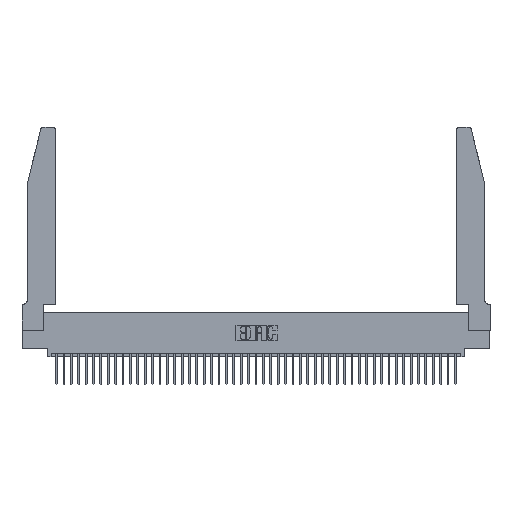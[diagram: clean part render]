
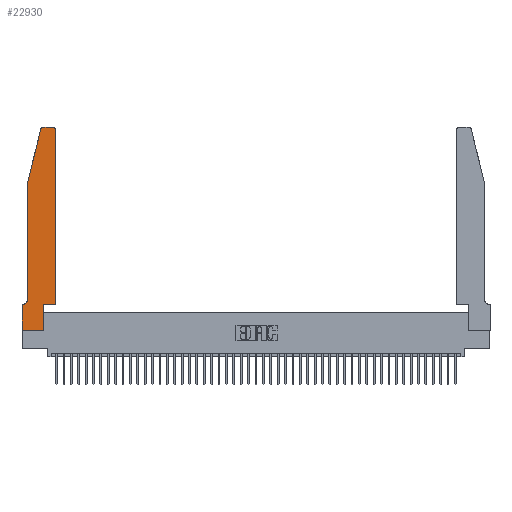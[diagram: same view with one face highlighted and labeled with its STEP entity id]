
A CAD part, top view. The second image highlights one B-rep face of the part: STEP entity #22930.
In plain terms, the highlighted planar face has unit normal (0, 0, 1).
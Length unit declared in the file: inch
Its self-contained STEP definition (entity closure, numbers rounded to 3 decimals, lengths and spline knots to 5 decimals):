
#414 = DIRECTION ( 'NONE',  ( 1., 0., 0. ) ) ;
#731 = VECTOR ( 'NONE', #16144, 39.37008 ) ;
#792 = CARTESIAN_POINT ( 'NONE',  ( 0., 0., 0.37 ) ) ;
#1232 = ORIENTED_EDGE ( 'NONE', *, *, #34104, .T. ) ;
#1706 = EDGE_CURVE ( 'NONE', #18084, #12142, #13387, .T. ) ;
#2321 = LINE ( 'NONE', #31248, #39360 ) ;
#2356 = VERTEX_POINT ( 'NONE', #45122 ) ;
#2507 = VECTOR ( 'NONE', #17822, 39.37008 ) ;
#2544 = DIRECTION ( 'NONE',  ( 0., 1., 0. ) ) ;
#3007 = DIRECTION ( 'NONE',  ( 0., 0., -1. ) ) ;
#3248 = VERTEX_POINT ( 'NONE', #18132 ) ;
#4471 = CARTESIAN_POINT ( 'NONE',  ( 0.0755, 2., 0.37 ) ) ;
#4486 = DIRECTION ( 'NONE',  ( 1., 0., 0. ) ) ;
#5032 = LINE ( 'NONE', #4471, #43030 ) ;
#5061 = DIRECTION ( 'NONE',  ( 0., 0., 1. ) ) ;
#5197 = VECTOR ( 'NONE', #2544, 39.37008 ) ;
#5380 = CARTESIAN_POINT ( 'NONE',  ( 0.0755, 0.42, 0.37 ) ) ;
#5472 = CIRCLE ( 'NONE', #22140, 0.07 ) ;
#6996 = VECTOR ( 'NONE', #44463, 39.37008 ) ;
#7797 = EDGE_CURVE ( 'NONE', #34003, #36792, #15695, .T. ) ;
#8155 = DIRECTION ( 'NONE',  ( 0., -1., 0. ) ) ;
#8232 = VERTEX_POINT ( 'NONE', #10209 ) ;
#9757 = CARTESIAN_POINT ( 'NONE',  ( 0.0755, 2., 0.37 ) ) ;
#9862 = CARTESIAN_POINT ( 'NONE',  ( 0., 0.35, 0.37 ) ) ;
#9913 = EDGE_CURVE ( 'NONE', #3248, #14087, #33858, .T. ) ;
#10167 = CARTESIAN_POINT ( 'NONE',  ( 0.4505, 2.72, 0.37 ) ) ;
#10209 = CARTESIAN_POINT ( 'NONE',  ( 0.2865, 0.35, 0.37 ) ) ;
#10376 = ORIENTED_EDGE ( 'NONE', *, *, #37209, .T. ) ;
#10499 = LINE ( 'NONE', #26812, #731 ) ;
#11829 = LINE ( 'NONE', #9757, #27554 ) ;
#12142 = VERTEX_POINT ( 'NONE', #45290 ) ;
#13387 = LINE ( 'NONE', #31409, #2507 ) ;
#13538 = DIRECTION ( 'NONE',  ( 1., 0., 0. ) ) ;
#14087 = VERTEX_POINT ( 'NONE', #10167 ) ;
#14396 = ORIENTED_EDGE ( 'NONE', *, *, #20613, .T. ) ;
#14770 = EDGE_CURVE ( 'NONE', #8232, #3248, #2321, .T. ) ;
#14876 = CARTESIAN_POINT ( 'NONE',  ( 0.2865, 0., 0.37 ) ) ;
#15167 = EDGE_LOOP ( 'NONE', ( #15466, #34423, #10376, #21123, #33890, #25610, #37212, #28919, #1232, #32279, #41601, #14396 ) ) ;
#15466 = ORIENTED_EDGE ( 'NONE', *, *, #33563, .T. ) ;
#15695 = LINE ( 'NONE', #792, #31376 ) ;
#16144 = DIRECTION ( 'NONE',  ( -1., 0., 0. ) ) ;
#17439 = DIRECTION ( 'NONE',  ( 0., -1., 0. ) ) ;
#17822 = DIRECTION ( 'NONE',  ( -1., 0., 0. ) ) ;
#17867 = AXIS2_PLACEMENT_3D ( 'NONE', #9862, #34877, #13538 ) ;
#18084 = VERTEX_POINT ( 'NONE', #20374 ) ;
#18132 = CARTESIAN_POINT ( 'NONE',  ( 0.4505, 0.35, 0.37 ) ) ;
#18966 = CARTESIAN_POINT ( 'NONE',  ( 0., 0., 0.37 ) ) ;
#19370 = CARTESIAN_POINT ( 'NONE',  ( 0.4205, 2.75, 0.37 ) ) ;
#19569 = CARTESIAN_POINT ( 'NONE',  ( 0.2865, 0.35, 0.37 ) ) ;
#19875 = AXIS2_PLACEMENT_3D ( 'NONE', #26706, #5061, #30272 ) ;
#20374 = CARTESIAN_POINT ( 'NONE',  ( 0.0055, 0.35, 0.37 ) ) ;
#20613 = EDGE_CURVE ( 'NONE', #14087, #37615, #25613, .T. ) ;
#21123 = ORIENTED_EDGE ( 'NONE', *, *, #28680, .T. ) ;
#22140 = AXIS2_PLACEMENT_3D ( 'NONE', #24723, #3007, #28285 ) ;
#22216 = DIRECTION ( 'NONE',  ( 0., 0., 1. ) ) ;
#22707 = FACE_OUTER_BOUND ( 'NONE', #15167, .T. ) ;
#22930 = ADVANCED_FACE ( 'NONE', ( #22707 ), #31381, .T. ) ;
#24165 = CIRCLE ( 'NONE', #19875, 0.03 ) ;
#24248 = DIRECTION ( 'NONE',  ( 1., 0., 0. ) ) ;
#24723 = CARTESIAN_POINT ( 'NONE',  ( 0.0055, 0.42, 0.37 ) ) ;
#25171 = EDGE_CURVE ( 'NONE', #25639, #18084, #5472, .T. ) ;
#25610 = ORIENTED_EDGE ( 'NONE', *, *, #1706, .T. ) ;
#25613 = CIRCLE ( 'NONE', #31285, 0.03 ) ;
#25639 = VERTEX_POINT ( 'NONE', #5380 ) ;
#26706 = CARTESIAN_POINT ( 'NONE',  ( 0.284, 2.72, 0.37 ) ) ;
#26812 = CARTESIAN_POINT ( 'NONE',  ( 0.2605, 2.75, 0.37 ) ) ;
#27554 = VECTOR ( 'NONE', #45360, 39.37008 ) ;
#28175 = VERTEX_POINT ( 'NONE', #30518 ) ;
#28285 = DIRECTION ( 'NONE',  ( -1., 0., 0. ) ) ;
#28680 = EDGE_CURVE ( 'NONE', #28175, #25639, #5032, .T. ) ;
#28919 = ORIENTED_EDGE ( 'NONE', *, *, #7797, .T. ) ;
#29690 = LINE ( 'NONE', #31951, #46134 ) ;
#30056 = EDGE_CURVE ( 'NONE', #33862, #2356, #24165, .T. ) ;
#30272 = DIRECTION ( 'NONE',  ( 1., 0., 0. ) ) ;
#30398 = EDGE_CURVE ( 'NONE', #12142, #34003, #29690, .T. ) ;
#30518 = CARTESIAN_POINT ( 'NONE',  ( 0.0755, 2., 0.37 ) ) ;
#31248 = CARTESIAN_POINT ( 'NONE',  ( 0.4505, 0.35, 0.37 ) ) ;
#31285 = AXIS2_PLACEMENT_3D ( 'NONE', #43341, #22216, #414 ) ;
#31376 = VECTOR ( 'NONE', #4486, 39.37008 ) ;
#31381 = PLANE ( 'NONE',  #17867 ) ;
#31409 = CARTESIAN_POINT ( 'NONE',  ( 0.0755, 0.35, 0.37 ) ) ;
#31951 = CARTESIAN_POINT ( 'NONE',  ( 0., 0., 0.37 ) ) ;
#32279 = ORIENTED_EDGE ( 'NONE', *, *, #14770, .T. ) ;
#33563 = EDGE_CURVE ( 'NONE', #37615, #33862, #10499, .T. ) ;
#33858 = LINE ( 'NONE', #41844, #5197 ) ;
#33862 = VERTEX_POINT ( 'NONE', #35580 ) ;
#33890 = ORIENTED_EDGE ( 'NONE', *, *, #25171, .T. ) ;
#34003 = VERTEX_POINT ( 'NONE', #18966 ) ;
#34104 = EDGE_CURVE ( 'NONE', #36792, #8232, #44915, .T. ) ;
#34423 = ORIENTED_EDGE ( 'NONE', *, *, #30056, .T. ) ;
#34877 = DIRECTION ( 'NONE',  ( 0., 0., 1. ) ) ;
#35580 = CARTESIAN_POINT ( 'NONE',  ( 0.284, 2.75, 0.37 ) ) ;
#36792 = VERTEX_POINT ( 'NONE', #14876 ) ;
#37209 = EDGE_CURVE ( 'NONE', #2356, #28175, #11829, .T. ) ;
#37212 = ORIENTED_EDGE ( 'NONE', *, *, #30398, .T. ) ;
#37615 = VERTEX_POINT ( 'NONE', #19370 ) ;
#39360 = VECTOR ( 'NONE', #24248, 39.37008 ) ;
#41601 = ORIENTED_EDGE ( 'NONE', *, *, #9913, .T. ) ;
#41844 = CARTESIAN_POINT ( 'NONE',  ( 0.4505, 0.35, 0.37 ) ) ;
#43030 = VECTOR ( 'NONE', #8155, 39.37008 ) ;
#43341 = CARTESIAN_POINT ( 'NONE',  ( 0.4205, 2.72, 0.37 ) ) ;
#44463 = DIRECTION ( 'NONE',  ( 0., 1., 0. ) ) ;
#44915 = LINE ( 'NONE', #19569, #6996 ) ;
#45122 = CARTESIAN_POINT ( 'NONE',  ( 0.25487, 2.72718, 0.37 ) ) ;
#45290 = CARTESIAN_POINT ( 'NONE',  ( 0., 0.35, 0.37 ) ) ;
#45360 = DIRECTION ( 'NONE',  ( -0.239, -0.971, 0. ) ) ;
#46134 = VECTOR ( 'NONE', #17439, 39.37008 ) ;
